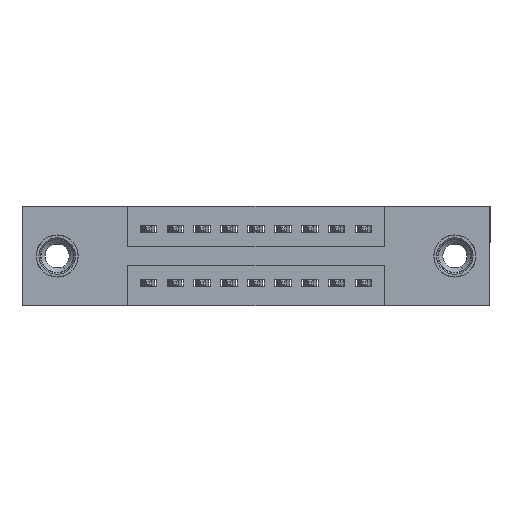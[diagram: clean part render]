
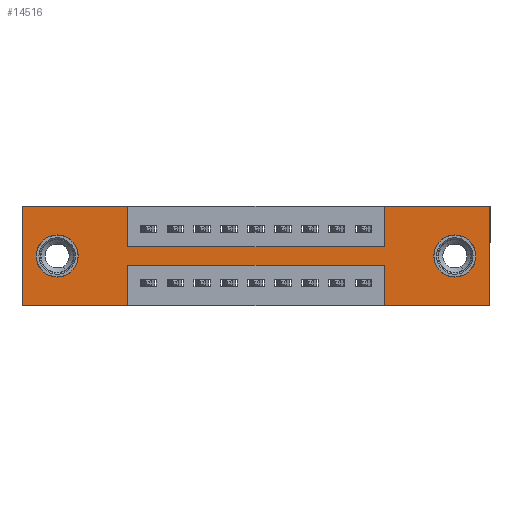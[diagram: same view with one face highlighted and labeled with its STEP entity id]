
A CAD part, front view. The second image highlights one B-rep face of the part: STEP entity #14516.
In plain terms, the highlighted planar face has unit normal (0, -1, 0).
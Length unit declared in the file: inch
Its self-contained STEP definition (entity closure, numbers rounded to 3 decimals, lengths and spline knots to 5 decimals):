
#28 = CARTESIAN_POINT ( 'NONE',  ( 1.605, 0., -0.263 ) ) ;
#143 = LINE ( 'NONE', #3386, #8785 ) ;
#150 = FACE_BOUND ( 'NONE', #15575, .T. ) ;
#159 = ORIENTED_EDGE ( 'NONE', *, *, #5277, .F. ) ;
#324 = VERTEX_POINT ( 'NONE', #556 ) ;
#556 = CARTESIAN_POINT ( 'NONE',  ( 1.3425, 0., 0. ) ) ;
#604 = DIRECTION ( 'NONE',  ( 1., 0., 0. ) ) ;
#787 = VERTEX_POINT ( 'NONE', #15713 ) ;
#816 = ORIENTED_EDGE ( 'NONE', *, *, #13324, .F. ) ;
#1315 = CARTESIAN_POINT ( 'NONE',  ( 0.3925, 0., 0. ) ) ;
#1426 = VERTEX_POINT ( 'NONE', #1907 ) ;
#1606 = VERTEX_POINT ( 'NONE', #2220 ) ;
#1740 = EDGE_CURVE ( 'NONE', #10876, #15203, #15802, .T. ) ;
#1782 = CARTESIAN_POINT ( 'NONE',  ( 0.3925, 0., -0.37 ) ) ;
#1876 = CARTESIAN_POINT ( 'NONE',  ( 1.3425, 0., -0.22 ) ) ;
#1900 = DIRECTION ( 'NONE',  ( 0., 0., 1. ) ) ;
#1907 = CARTESIAN_POINT ( 'NONE',  ( 1.735, 0., -0.37 ) ) ;
#1986 = AXIS2_PLACEMENT_3D ( 'NONE', #5390, #15554, #6739 ) ;
#1994 = CARTESIAN_POINT ( 'NONE',  ( 1.605, 0., -0.185 ) ) ;
#2062 = ORIENTED_EDGE ( 'NONE', *, *, #13062, .F. ) ;
#2220 = CARTESIAN_POINT ( 'NONE',  ( 0.13, 0., -0.107 ) ) ;
#2289 = CARTESIAN_POINT ( 'NONE',  ( 0., 0., 0. ) ) ;
#2390 = VERTEX_POINT ( 'NONE', #12183 ) ;
#2536 = LINE ( 'NONE', #1782, #3513 ) ;
#2890 = DIRECTION ( 'NONE',  ( 0., 0., -1. ) ) ;
#2924 = AXIS2_PLACEMENT_3D ( 'NONE', #13432, #8261, #10846 ) ;
#2948 = VERTEX_POINT ( 'NONE', #11920 ) ;
#3067 = CARTESIAN_POINT ( 'NONE',  ( 1.3425, 0., -0.37 ) ) ;
#3121 = DIRECTION ( 'NONE',  ( 0., 0., -1. ) ) ;
#3175 = PLANE ( 'NONE',  #10520 ) ;
#3211 = CARTESIAN_POINT ( 'NONE',  ( 0., 0., 0. ) ) ;
#3249 = DIRECTION ( 'NONE',  ( 0., 0., -1. ) ) ;
#3312 = VERTEX_POINT ( 'NONE', #6476 ) ;
#3386 = CARTESIAN_POINT ( 'NONE',  ( 0., 0., -0.37 ) ) ;
#3391 = ORIENTED_EDGE ( 'NONE', *, *, #15758, .F. ) ;
#3513 = VECTOR ( 'NONE', #13077, 39.37008 ) ;
#3543 = ORIENTED_EDGE ( 'NONE', *, *, #10785, .T. ) ;
#3643 = EDGE_CURVE ( 'NONE', #7589, #16093, #15151, .T. ) ;
#3704 = VERTEX_POINT ( 'NONE', #28 ) ;
#3771 = VECTOR ( 'NONE', #14727, 39.37008 ) ;
#4220 = ORIENTED_EDGE ( 'NONE', *, *, #14143, .F. ) ;
#4404 = CARTESIAN_POINT ( 'NONE',  ( 0.3925, 0., -0.15 ) ) ;
#4534 = ORIENTED_EDGE ( 'NONE', *, *, #11170, .F. ) ;
#4630 = LINE ( 'NONE', #10406, #15443 ) ;
#4707 = ORIENTED_EDGE ( 'NONE', *, *, #6718, .T. ) ;
#4886 = VERTEX_POINT ( 'NONE', #5713 ) ;
#4907 = LINE ( 'NONE', #1315, #11147 ) ;
#5137 = AXIS2_PLACEMENT_3D ( 'NONE', #1994, #10762, #3249 ) ;
#5277 = EDGE_CURVE ( 'NONE', #2390, #324, #15093, .T. ) ;
#5390 = CARTESIAN_POINT ( 'NONE',  ( 0.13, 0., -0.185 ) ) ;
#5713 = CARTESIAN_POINT ( 'NONE',  ( 0.3925, 0., -0.37 ) ) ;
#6182 = CARTESIAN_POINT ( 'NONE',  ( 0.3925, 0., 0. ) ) ;
#6188 = CARTESIAN_POINT ( 'NONE',  ( 0., 0., 0. ) ) ;
#6194 = ORIENTED_EDGE ( 'NONE', *, *, #10244, .F. ) ;
#6238 = EDGE_CURVE ( 'NONE', #3704, #15603, #14495, .T. ) ;
#6273 = ORIENTED_EDGE ( 'NONE', *, *, #15299, .F. ) ;
#6476 = CARTESIAN_POINT ( 'NONE',  ( 0., 0., -0.37 ) ) ;
#6651 = VERTEX_POINT ( 'NONE', #13383 ) ;
#6714 = ORIENTED_EDGE ( 'NONE', *, *, #10448, .T. ) ;
#6718 = EDGE_CURVE ( 'NONE', #15603, #3704, #10545, .T. ) ;
#6739 = DIRECTION ( 'NONE',  ( 0., 0., 1. ) ) ;
#6851 = EDGE_LOOP ( 'NONE', ( #3543, #6714 ) ) ;
#6876 = CARTESIAN_POINT ( 'NONE',  ( 1.3425, 0., 0. ) ) ;
#6969 = DIRECTION ( 'NONE',  ( 1., 0., 0. ) ) ;
#6982 = LINE ( 'NONE', #2289, #7962 ) ;
#6998 = LINE ( 'NONE', #3067, #10556 ) ;
#7526 = DIRECTION ( 'NONE',  ( -1., 0., 0. ) ) ;
#7589 = VERTEX_POINT ( 'NONE', #6188 ) ;
#7653 = CARTESIAN_POINT ( 'NONE',  ( 1.605, 0., -0.107 ) ) ;
#7962 = VECTOR ( 'NONE', #8582, 39.37008 ) ;
#7998 = VECTOR ( 'NONE', #1900, 39.37008 ) ;
#8215 = LINE ( 'NONE', #4404, #12352 ) ;
#8261 = DIRECTION ( 'NONE',  ( 0., 1., 0. ) ) ;
#8582 = DIRECTION ( 'NONE',  ( 0., 0., 1. ) ) ;
#8681 = CARTESIAN_POINT ( 'NONE',  ( 0.13, 0., -0.185 ) ) ;
#8785 = VECTOR ( 'NONE', #9734, 39.37008 ) ;
#9112 = ORIENTED_EDGE ( 'NONE', *, *, #3643, .F. ) ;
#9623 = VECTOR ( 'NONE', #10854, 39.37008 ) ;
#9701 = CARTESIAN_POINT ( 'NONE',  ( 0., 0., -0.37 ) ) ;
#9734 = DIRECTION ( 'NONE',  ( -1., 0., 0. ) ) ;
#10244 = EDGE_CURVE ( 'NONE', #324, #2948, #14995, .T. ) ;
#10388 = AXIS2_PLACEMENT_3D ( 'NONE', #8681, #14955, #13574 ) ;
#10406 = CARTESIAN_POINT ( 'NONE',  ( 1.735, 0., 0. ) ) ;
#10448 = EDGE_CURVE ( 'NONE', #13728, #1606, #12992, .T. ) ;
#10520 = AXIS2_PLACEMENT_3D ( 'NONE', #12002, #12994, #3121 ) ;
#10545 = CIRCLE ( 'NONE', #2924, 0.078 ) ;
#10556 = VECTOR ( 'NONE', #11844, 39.37008 ) ;
#10762 = DIRECTION ( 'NONE',  ( 0., 1., 0. ) ) ;
#10785 = EDGE_CURVE ( 'NONE', #1606, #13728, #12195, .T. ) ;
#10846 = DIRECTION ( 'NONE',  ( 0., 0., -1. ) ) ;
#10854 = DIRECTION ( 'NONE',  ( 1., 0., 0. ) ) ;
#10876 = VERTEX_POINT ( 'NONE', #1876 ) ;
#10908 = ORIENTED_EDGE ( 'NONE', *, *, #14596, .F. ) ;
#11126 = FACE_BOUND ( 'NONE', #6851, .T. ) ;
#11147 = VECTOR ( 'NONE', #11289, 39.37008 ) ;
#11170 = EDGE_CURVE ( 'NONE', #4886, #3312, #13182, .T. ) ;
#11289 = DIRECTION ( 'NONE',  ( 0., 0., -1. ) ) ;
#11312 = CARTESIAN_POINT ( 'NONE',  ( 0.3925, 0., -0.22 ) ) ;
#11427 = VECTOR ( 'NONE', #6969, 39.37008 ) ;
#11592 = ORIENTED_EDGE ( 'NONE', *, *, #6238, .T. ) ;
#11844 = DIRECTION ( 'NONE',  ( 0., 0., 1. ) ) ;
#11920 = CARTESIAN_POINT ( 'NONE',  ( 1.735, 0., 0. ) ) ;
#12002 = CARTESIAN_POINT ( 'NONE',  ( 0., 0., -0.37 ) ) ;
#12161 = CARTESIAN_POINT ( 'NONE',  ( 0., 0., 0. ) ) ;
#12183 = CARTESIAN_POINT ( 'NONE',  ( 1.3425, 0., -0.15 ) ) ;
#12195 = CIRCLE ( 'NONE', #1986, 0.078 ) ;
#12352 = VECTOR ( 'NONE', #604, 39.37008 ) ;
#12409 = EDGE_LOOP ( 'NONE', ( #816, #13694, #10908, #4220, #3391, #6194, #159, #2062, #14111, #9112, #6273, #4534 ) ) ;
#12992 = CIRCLE ( 'NONE', #10388, 0.078 ) ;
#12994 = DIRECTION ( 'NONE',  ( 0., -1., 0. ) ) ;
#13062 = EDGE_CURVE ( 'NONE', #6651, #2390, #8215, .T. ) ;
#13077 = DIRECTION ( 'NONE',  ( 0., 0., -1. ) ) ;
#13182 = LINE ( 'NONE', #9701, #3771 ) ;
#13324 = EDGE_CURVE ( 'NONE', #15203, #4886, #2536, .T. ) ;
#13383 = CARTESIAN_POINT ( 'NONE',  ( 0.3925, 0., -0.15 ) ) ;
#13432 = CARTESIAN_POINT ( 'NONE',  ( 1.605, 0., -0.185 ) ) ;
#13574 = DIRECTION ( 'NONE',  ( 0., 0., 1. ) ) ;
#13694 = ORIENTED_EDGE ( 'NONE', *, *, #1740, .F. ) ;
#13728 = VERTEX_POINT ( 'NONE', #15794 ) ;
#14100 = FACE_OUTER_BOUND ( 'NONE', #12409, .T. ) ;
#14111 = ORIENTED_EDGE ( 'NONE', *, *, #14290, .F. ) ;
#14143 = EDGE_CURVE ( 'NONE', #1426, #787, #143, .T. ) ;
#14265 = CARTESIAN_POINT ( 'NONE',  ( 0.3925, 0., -0.22 ) ) ;
#14290 = EDGE_CURVE ( 'NONE', #16093, #6651, #4907, .T. ) ;
#14495 = CIRCLE ( 'NONE', #5137, 0.078 ) ;
#14516 = ADVANCED_FACE ( 'NONE', ( #150, #11126, #14100 ), #3175, .T. ) ;
#14596 = EDGE_CURVE ( 'NONE', #787, #10876, #6998, .T. ) ;
#14727 = DIRECTION ( 'NONE',  ( -1., 0., 0. ) ) ;
#14955 = DIRECTION ( 'NONE',  ( 0., 1., 0. ) ) ;
#14995 = LINE ( 'NONE', #3211, #11427 ) ;
#15093 = LINE ( 'NONE', #6876, #7998 ) ;
#15151 = LINE ( 'NONE', #12161, #9623 ) ;
#15203 = VERTEX_POINT ( 'NONE', #14265 ) ;
#15299 = EDGE_CURVE ( 'NONE', #3312, #7589, #6982, .T. ) ;
#15413 = VECTOR ( 'NONE', #7526, 39.37008 ) ;
#15443 = VECTOR ( 'NONE', #2890, 39.37008 ) ;
#15554 = DIRECTION ( 'NONE',  ( 0., 1., 0. ) ) ;
#15575 = EDGE_LOOP ( 'NONE', ( #4707, #11592 ) ) ;
#15603 = VERTEX_POINT ( 'NONE', #7653 ) ;
#15713 = CARTESIAN_POINT ( 'NONE',  ( 1.3425, 0., -0.37 ) ) ;
#15758 = EDGE_CURVE ( 'NONE', #2948, #1426, #4630, .T. ) ;
#15794 = CARTESIAN_POINT ( 'NONE',  ( 0.13, 0., -0.263 ) ) ;
#15802 = LINE ( 'NONE', #11312, #15413 ) ;
#16093 = VERTEX_POINT ( 'NONE', #6182 ) ;
